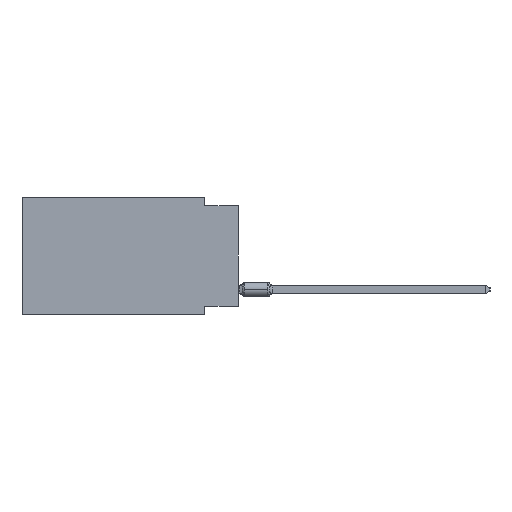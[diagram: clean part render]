
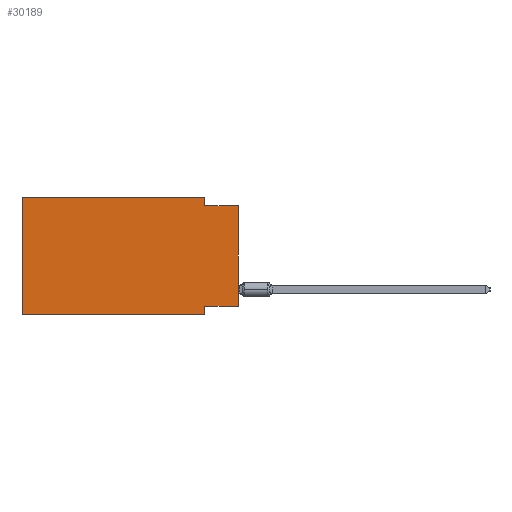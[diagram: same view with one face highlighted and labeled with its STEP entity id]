
A CAD part, left-side view. The second image highlights one B-rep face of the part: STEP entity #30189.
In plain terms, the highlighted planar face has unit normal (-1, 0, 0).
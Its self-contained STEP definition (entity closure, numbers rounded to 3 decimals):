
#602 = DIRECTION ( 'NONE',  ( 0., 0., 1. ) ) ;
#1350 = FACE_OUTER_BOUND ( 'NONE', #55049, .T. ) ;
#1574 = DIRECTION ( 'NONE',  ( 0., 0., 1. ) ) ;
#3673 = EDGE_CURVE ( 'NONE', #37016, #5642, #51361, .T. ) ;
#4401 = DIRECTION ( 'NONE',  ( 0., -1., 0. ) ) ;
#4585 = VECTOR ( 'NONE', #33834, 1000. ) ;
#4803 = ORIENTED_EDGE ( 'NONE', *, *, #32874, .T. ) ;
#5642 = VERTEX_POINT ( 'NONE', #41603 ) ;
#6141 = DIRECTION ( 'NONE',  ( 0., 0., -1. ) ) ;
#7545 = CARTESIAN_POINT ( 'NONE',  ( 0., 16.383, 0. ) ) ;
#7835 = CARTESIAN_POINT ( 'NONE',  ( 0., 2.54, -0.635 ) ) ;
#8716 = ORIENTED_EDGE ( 'NONE', *, *, #56092, .F. ) ;
#10980 = VECTOR ( 'NONE', #32452, 1000. ) ;
#12491 = EDGE_CURVE ( 'NONE', #55248, #37016, #39689, .T. ) ;
#13503 = CARTESIAN_POINT ( 'NONE',  ( 0., 16.383, -8.89 ) ) ;
#14016 = EDGE_CURVE ( 'NONE', #56084, #23153, #52325, .T. ) ;
#14080 = VERTEX_POINT ( 'NONE', #40243 ) ;
#14285 = VERTEX_POINT ( 'NONE', #41377 ) ;
#14936 = LINE ( 'NONE', #49114, #10980 ) ;
#15688 = ORIENTED_EDGE ( 'NONE', *, *, #21580, .T. ) ;
#16312 = CARTESIAN_POINT ( 'NONE',  ( 0., 16.383, 0. ) ) ;
#20941 = LINE ( 'NONE', #47924, #32135 ) ;
#21060 = EDGE_CURVE ( 'NONE', #5642, #47072, #14936, .T. ) ;
#21578 = VECTOR ( 'NONE', #1574, 1000. ) ;
#21580 = EDGE_CURVE ( 'NONE', #55248, #14080, #20941, .T. ) ;
#23153 = VERTEX_POINT ( 'NONE', #45596 ) ;
#23461 = CARTESIAN_POINT ( 'NONE',  ( 0., 16.383, 0. ) ) ;
#25643 = CARTESIAN_POINT ( 'NONE',  ( 0., 0., -8.255 ) ) ;
#27984 = CARTESIAN_POINT ( 'NONE',  ( 0., 2.54, -8.89 ) ) ;
#30189 = ADVANCED_FACE ( 'NONE', ( #1350 ), #40704, .F. ) ;
#31995 = ORIENTED_EDGE ( 'NONE', *, *, #12491, .F. ) ;
#32135 = VECTOR ( 'NONE', #43619, 1000. ) ;
#32452 = DIRECTION ( 'NONE',  ( 0., 0., -1. ) ) ;
#32874 = EDGE_CURVE ( 'NONE', #56084, #14285, #53285, .T. ) ;
#33834 = DIRECTION ( 'NONE',  ( 0., -1., 0. ) ) ;
#36023 = LINE ( 'NONE', #27984, #40215 ) ;
#37016 = VERTEX_POINT ( 'NONE', #7545 ) ;
#39689 = LINE ( 'NONE', #39962, #49836 ) ;
#39962 = CARTESIAN_POINT ( 'NONE',  ( 0., 16.383, 0. ) ) ;
#40215 = VECTOR ( 'NONE', #6141, 1000. ) ;
#40243 = CARTESIAN_POINT ( 'NONE',  ( 0., 2.54, -8.89 ) ) ;
#40704 = PLANE ( 'NONE',  #50805 ) ;
#41377 = CARTESIAN_POINT ( 'NONE',  ( 0., 0., -0.635 ) ) ;
#41603 = CARTESIAN_POINT ( 'NONE',  ( 0., 2.54, 0. ) ) ;
#43619 = DIRECTION ( 'NONE',  ( 0., -1., 0. ) ) ;
#44047 = CARTESIAN_POINT ( 'NONE',  ( 0., 0., -0.635 ) ) ;
#44783 = VECTOR ( 'NONE', #4401, 1000. ) ;
#45133 = ORIENTED_EDGE ( 'NONE', *, *, #21060, .F. ) ;
#45596 = CARTESIAN_POINT ( 'NONE',  ( 0., 2.54, -8.255 ) ) ;
#46149 = DIRECTION ( 'NONE',  ( 0., 0., -1. ) ) ;
#47072 = VERTEX_POINT ( 'NONE', #7835 ) ;
#47456 = DIRECTION ( 'NONE',  ( 0., 1., 0. ) ) ;
#47924 = CARTESIAN_POINT ( 'NONE',  ( 0., 16.383, -8.89 ) ) ;
#48816 = ORIENTED_EDGE ( 'NONE', *, *, #52584, .F. ) ;
#48945 = CARTESIAN_POINT ( 'NONE',  ( 0., 0., -8.255 ) ) ;
#49114 = CARTESIAN_POINT ( 'NONE',  ( 0., 2.54, 0. ) ) ;
#49836 = VECTOR ( 'NONE', #602, 1000. ) ;
#50805 = AXIS2_PLACEMENT_3D ( 'NONE', #23461, #54746, #46149 ) ;
#51361 = LINE ( 'NONE', #16312, #4585 ) ;
#52325 = LINE ( 'NONE', #25643, #52734 ) ;
#52584 = EDGE_CURVE ( 'NONE', #47072, #14285, #52915, .T. ) ;
#52734 = VECTOR ( 'NONE', #47456, 1000. ) ;
#52915 = LINE ( 'NONE', #44047, #44783 ) ;
#53285 = LINE ( 'NONE', #53839, #21578 ) ;
#53839 = CARTESIAN_POINT ( 'NONE',  ( 0., 0., 0. ) ) ;
#54107 = ORIENTED_EDGE ( 'NONE', *, *, #14016, .F. ) ;
#54746 = DIRECTION ( 'NONE',  ( 1., 0., 0. ) ) ;
#55049 = EDGE_LOOP ( 'NONE', ( #4803, #48816, #45133, #56811, #31995, #15688, #8716, #54107 ) ) ;
#55248 = VERTEX_POINT ( 'NONE', #13503 ) ;
#56084 = VERTEX_POINT ( 'NONE', #48945 ) ;
#56092 = EDGE_CURVE ( 'NONE', #23153, #14080, #36023, .T. ) ;
#56811 = ORIENTED_EDGE ( 'NONE', *, *, #3673, .F. ) ;
